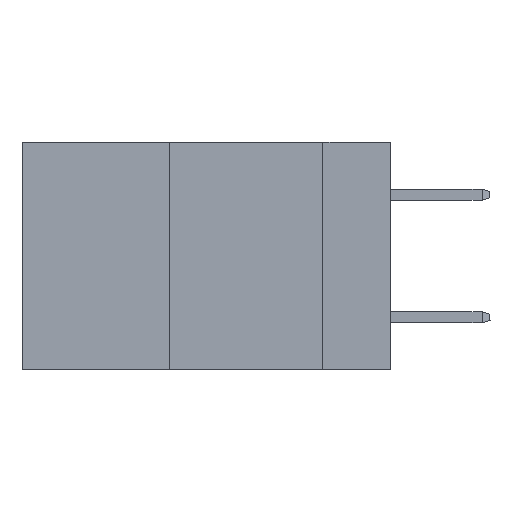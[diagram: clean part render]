
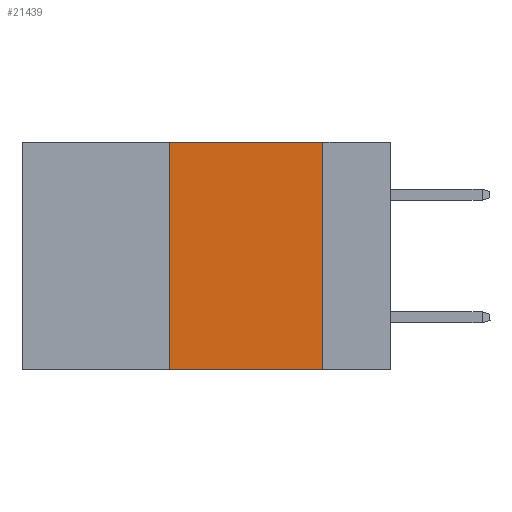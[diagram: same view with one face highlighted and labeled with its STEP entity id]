
A CAD part, left-side view. The second image highlights one B-rep face of the part: STEP entity #21439.
In plain terms, the highlighted planar face has unit normal (-1, 0, 0).
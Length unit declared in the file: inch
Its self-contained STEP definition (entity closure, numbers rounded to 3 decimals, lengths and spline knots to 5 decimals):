
#890 = VECTOR ( 'NONE', #9008, 39.37008 ) ;
#1166 = CARTESIAN_POINT ( 'NONE',  ( 0., 0.6, 0. ) ) ;
#1637 = ORIENTED_EDGE ( 'NONE', *, *, #22539, .F. ) ;
#1916 = LINE ( 'NONE', #17481, #2596 ) ;
#2596 = VECTOR ( 'NONE', #21879, 39.37008 ) ;
#2837 = VERTEX_POINT ( 'NONE', #8762 ) ;
#3902 = CARTESIAN_POINT ( 'NONE',  ( 0., 0.11, -0.37 ) ) ;
#6032 = LINE ( 'NONE', #15712, #21948 ) ;
#6843 = AXIS2_PLACEMENT_3D ( 'NONE', #1166, #12445, #16868 ) ;
#8762 = CARTESIAN_POINT ( 'NONE',  ( 0., 0.11, 0. ) ) ;
#9008 = DIRECTION ( 'NONE',  ( 0., -1., 0. ) ) ;
#9043 = DIRECTION ( 'NONE',  ( 0., 0., -1. ) ) ;
#10207 = EDGE_CURVE ( 'NONE', #16523, #2837, #16733, .T. ) ;
#11032 = CARTESIAN_POINT ( 'NONE',  ( 0., 0.36, -0.37 ) ) ;
#11292 = DIRECTION ( 'NONE',  ( 0., 0., 1. ) ) ;
#11854 = VERTEX_POINT ( 'NONE', #11032 ) ;
#12445 = DIRECTION ( 'NONE',  ( 1., 0., 0. ) ) ;
#13351 = CARTESIAN_POINT ( 'NONE',  ( 0., 0.6, 0. ) ) ;
#13770 = VECTOR ( 'NONE', #9043, 39.37008 ) ;
#13821 = FACE_OUTER_BOUND ( 'NONE', #26024, .T. ) ;
#15122 = EDGE_CURVE ( 'NONE', #11854, #16523, #6032, .T. ) ;
#15712 = CARTESIAN_POINT ( 'NONE',  ( 0., 0.36, 0. ) ) ;
#16523 = VERTEX_POINT ( 'NONE', #21444 ) ;
#16574 = PLANE ( 'NONE',  #6843 ) ;
#16733 = LINE ( 'NONE', #13351, #890 ) ;
#16868 = DIRECTION ( 'NONE',  ( 0., 0., -1. ) ) ;
#17481 = CARTESIAN_POINT ( 'NONE',  ( 0., 0.6, -0.37 ) ) ;
#17633 = ORIENTED_EDGE ( 'NONE', *, *, #10207, .F. ) ;
#18398 = VERTEX_POINT ( 'NONE', #3902 ) ;
#18460 = EDGE_CURVE ( 'NONE', #11854, #18398, #1916, .T. ) ;
#20445 = CARTESIAN_POINT ( 'NONE',  ( 0., 0.11, 0. ) ) ;
#20703 = LINE ( 'NONE', #20445, #13770 ) ;
#21439 = ADVANCED_FACE ( 'NONE', ( #13821 ), #16574, .F. ) ;
#21444 = CARTESIAN_POINT ( 'NONE',  ( 0., 0.36, 0. ) ) ;
#21879 = DIRECTION ( 'NONE',  ( 0., -1., 0. ) ) ;
#21948 = VECTOR ( 'NONE', #11292, 39.37008 ) ;
#22539 = EDGE_CURVE ( 'NONE', #2837, #18398, #20703, .T. ) ;
#26024 = EDGE_LOOP ( 'NONE', ( #1637, #17633, #27231, #28290 ) ) ;
#27231 = ORIENTED_EDGE ( 'NONE', *, *, #15122, .F. ) ;
#28290 = ORIENTED_EDGE ( 'NONE', *, *, #18460, .T. ) ;
